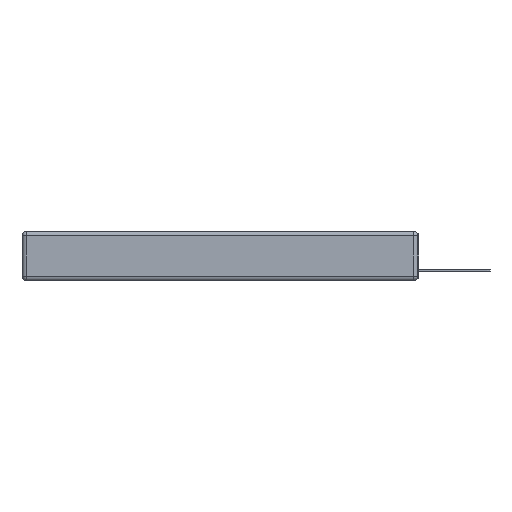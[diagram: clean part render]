
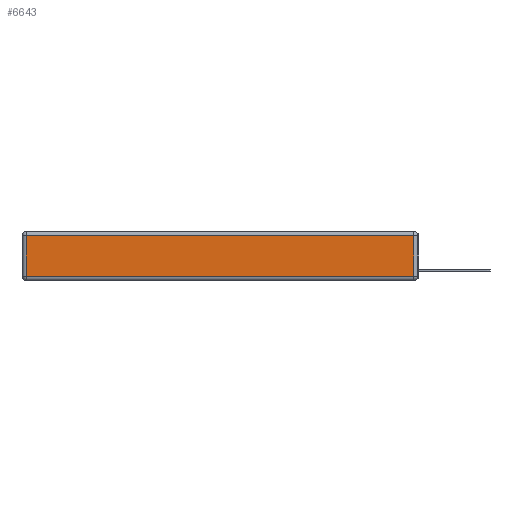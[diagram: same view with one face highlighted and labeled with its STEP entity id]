
A CAD part, left-side view. The second image highlights one B-rep face of the part: STEP entity #6643.
In plain terms, the highlighted planar face has unit normal (-1, 0, 0).
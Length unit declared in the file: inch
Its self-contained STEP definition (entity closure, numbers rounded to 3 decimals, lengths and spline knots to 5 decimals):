
#486 = FACE_OUTER_BOUND ( 'NONE', #16578, .T. ) ;
#3178 = VERTEX_POINT ( 'NONE', #15128 ) ;
#5214 = VERTEX_POINT ( 'NONE', #23999 ) ;
#6156 = VERTEX_POINT ( 'NONE', #14161 ) ;
#6388 = EDGE_CURVE ( 'NONE', #6156, #3178, #22042, .T. ) ;
#6590 = VECTOR ( 'NONE', #16088, 39.37008 ) ;
#6643 = ADVANCED_FACE ( 'NONE', ( #486 ), #8875, .T. ) ;
#6665 = AXIS2_PLACEMENT_3D ( 'NONE', #19796, #23612, #23765 ) ;
#7032 = CARTESIAN_POINT ( 'NONE',  ( 0., 0.03, -0.343 ) ) ;
#8035 = VECTOR ( 'NONE', #18272, 39.37008 ) ;
#8875 = PLANE ( 'NONE',  #6665 ) ;
#9192 = VECTOR ( 'NONE', #15885, 39.37008 ) ;
#9367 = EDGE_CURVE ( 'NONE', #11089, #5214, #19114, .T. ) ;
#10215 = EDGE_CURVE ( 'NONE', #3178, #11089, #10350, .T. ) ;
#10350 = LINE ( 'NONE', #23058, #9192 ) ;
#11089 = VERTEX_POINT ( 'NONE', #24011 ) ;
#11352 = ORIENTED_EDGE ( 'NONE', *, *, #10215, .T. ) ;
#13464 = ORIENTED_EDGE ( 'NONE', *, *, #9367, .T. ) ;
#14161 = CARTESIAN_POINT ( 'NONE',  ( 0., 2.72, -0.03 ) ) ;
#15128 = CARTESIAN_POINT ( 'NONE',  ( 0., 2.72, -0.313 ) ) ;
#15885 = DIRECTION ( 'NONE',  ( 0., -1., 0. ) ) ;
#16088 = DIRECTION ( 'NONE',  ( 0., 0., -1. ) ) ;
#16578 = EDGE_LOOP ( 'NONE', ( #11352, #13464, #19733, #21745 ) ) ;
#16767 = LINE ( 'NONE', #20529, #22889 ) ;
#18272 = DIRECTION ( 'NONE',  ( 0., 0., 1. ) ) ;
#19114 = LINE ( 'NONE', #7032, #8035 ) ;
#19286 = EDGE_CURVE ( 'NONE', #5214, #6156, #16767, .T. ) ;
#19733 = ORIENTED_EDGE ( 'NONE', *, *, #19286, .T. ) ;
#19762 = CARTESIAN_POINT ( 'NONE',  ( 0., 2.72, -0.343 ) ) ;
#19796 = CARTESIAN_POINT ( 'NONE',  ( 0., 0., -0.343 ) ) ;
#20529 = CARTESIAN_POINT ( 'NONE',  ( 0., 2.75, -0.03 ) ) ;
#20775 = DIRECTION ( 'NONE',  ( 0., 1., 0. ) ) ;
#21745 = ORIENTED_EDGE ( 'NONE', *, *, #6388, .T. ) ;
#22042 = LINE ( 'NONE', #19762, #6590 ) ;
#22889 = VECTOR ( 'NONE', #20775, 39.37008 ) ;
#23058 = CARTESIAN_POINT ( 'NONE',  ( 0., 0., -0.313 ) ) ;
#23612 = DIRECTION ( 'NONE',  ( -1., 0., 0. ) ) ;
#23765 = DIRECTION ( 'NONE',  ( 0., 0., 1. ) ) ;
#23999 = CARTESIAN_POINT ( 'NONE',  ( 0., 0.03, -0.03 ) ) ;
#24011 = CARTESIAN_POINT ( 'NONE',  ( 0., 0.03, -0.313 ) ) ;
